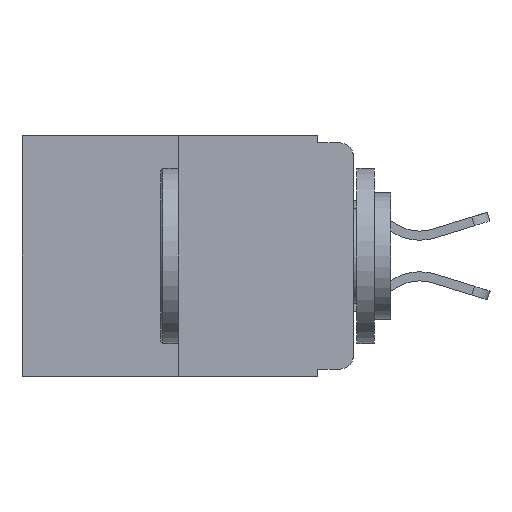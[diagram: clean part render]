
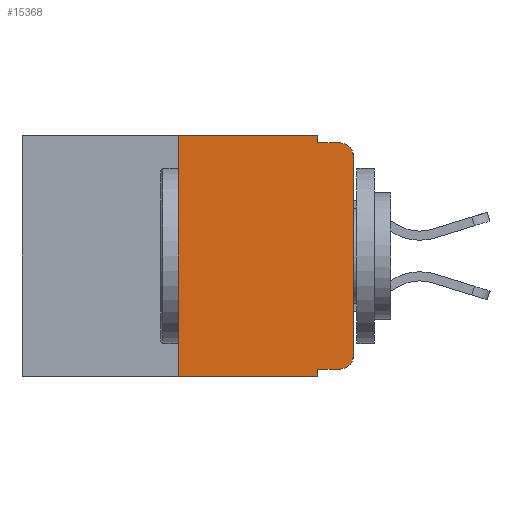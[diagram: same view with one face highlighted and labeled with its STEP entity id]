
A CAD part, left-side view. The second image highlights one B-rep face of the part: STEP entity #15368.
In plain terms, the highlighted planar face has unit normal (-1, 0, 0).
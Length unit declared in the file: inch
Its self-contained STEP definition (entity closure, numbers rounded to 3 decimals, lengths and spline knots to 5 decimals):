
#234 = ORIENTED_EDGE ( 'NONE', *, *, #13772, .T. ) ;
#562 = CARTESIAN_POINT ( 'NONE',  ( 0., 0.02, -0.03 ) ) ;
#959 = ORIENTED_EDGE ( 'NONE', *, *, #2726, .T. ) ;
#1015 = ORIENTED_EDGE ( 'NONE', *, *, #2249, .F. ) ;
#1059 = LINE ( 'NONE', #11792, #5077 ) ;
#1113 = CARTESIAN_POINT ( 'NONE',  ( 0., 0.25, 0. ) ) ;
#1494 = EDGE_LOOP ( 'NONE', ( #15183, #959, #10539, #1015, #7607, #7283, #234, #2650, #3972, #12098 ) ) ;
#1776 = VECTOR ( 'NONE', #1814, 39.37008 ) ;
#1783 = CARTESIAN_POINT ( 'NONE',  ( 0., 0.25, 0. ) ) ;
#1814 = DIRECTION ( 'NONE',  ( 0., 0., -1. ) ) ;
#2084 = LINE ( 'NONE', #13075, #10137 ) ;
#2249 = EDGE_CURVE ( 'NONE', #5030, #8816, #14380, .T. ) ;
#2281 = AXIS2_PLACEMENT_3D ( 'NONE', #12728, #11299, #8913 ) ;
#2309 = VERTEX_POINT ( 'NONE', #2767 ) ;
#2650 = ORIENTED_EDGE ( 'NONE', *, *, #3902, .F. ) ;
#2726 = EDGE_CURVE ( 'NONE', #13421, #11407, #7507, .T. ) ;
#2767 = CARTESIAN_POINT ( 'NONE',  ( 0., 0.25, -0.343 ) ) ;
#2811 = CARTESIAN_POINT ( 'NONE',  ( 0., 0., -0.03 ) ) ;
#2912 = CARTESIAN_POINT ( 'NONE',  ( 0., 0., -0.313 ) ) ;
#3123 = VERTEX_POINT ( 'NONE', #8086 ) ;
#3195 = VECTOR ( 'NONE', #13017, 39.37008 ) ;
#3245 = CARTESIAN_POINT ( 'NONE',  ( 0., 0.051, 0. ) ) ;
#3513 = CIRCLE ( 'NONE', #2281, 0.02 ) ;
#3902 = EDGE_CURVE ( 'NONE', #3123, #12696, #7713, .T. ) ;
#3972 = ORIENTED_EDGE ( 'NONE', *, *, #10650, .T. ) ;
#3991 = EDGE_CURVE ( 'NONE', #5268, #13049, #3513, .T. ) ;
#4136 = DIRECTION ( 'NONE',  ( -1., 0., 0. ) ) ;
#4153 = CARTESIAN_POINT ( 'NONE',  ( 0., 0.051, 0. ) ) ;
#4426 = CARTESIAN_POINT ( 'NONE',  ( 0., 0.473, -0.343 ) ) ;
#4637 = DIRECTION ( 'NONE',  ( 0., -1., 0. ) ) ;
#5030 = VERTEX_POINT ( 'NONE', #7222 ) ;
#5077 = VECTOR ( 'NONE', #4637, 39.37008 ) ;
#5268 = VERTEX_POINT ( 'NONE', #6978 ) ;
#5387 = CARTESIAN_POINT ( 'NONE',  ( 0., 0.051, -0.333 ) ) ;
#5455 = LINE ( 'NONE', #5387, #13763 ) ;
#5885 = DIRECTION ( 'NONE',  ( 0., 0., 1. ) ) ;
#6843 = CARTESIAN_POINT ( 'NONE',  ( 0., 0.051, -0.343 ) ) ;
#6978 = CARTESIAN_POINT ( 'NONE',  ( 0., 0.02, -0.333 ) ) ;
#7222 = CARTESIAN_POINT ( 'NONE',  ( 0., 0.051, 0. ) ) ;
#7283 = ORIENTED_EDGE ( 'NONE', *, *, #11773, .F. ) ;
#7507 = CIRCLE ( 'NONE', #9038, 0.02 ) ;
#7607 = ORIENTED_EDGE ( 'NONE', *, *, #8214, .F. ) ;
#7713 = LINE ( 'NONE', #4153, #1776 ) ;
#7765 = DIRECTION ( 'NONE',  ( 0., -1., 0. ) ) ;
#8025 = DIRECTION ( 'NONE',  ( 0., -1., 0. ) ) ;
#8056 = VERTEX_POINT ( 'NONE', #1783 ) ;
#8086 = CARTESIAN_POINT ( 'NONE',  ( 0., 0.051, -0.333 ) ) ;
#8108 = AXIS2_PLACEMENT_3D ( 'NONE', #8296, #13148, #10676 ) ;
#8214 = EDGE_CURVE ( 'NONE', #8056, #5030, #1059, .T. ) ;
#8296 = CARTESIAN_POINT ( 'NONE',  ( 0., 0.473, 0. ) ) ;
#8583 = CARTESIAN_POINT ( 'NONE',  ( 0., 0.051, -0.01 ) ) ;
#8816 = VERTEX_POINT ( 'NONE', #8583 ) ;
#8913 = DIRECTION ( 'NONE',  ( 0., 0., -1. ) ) ;
#8967 = VECTOR ( 'NONE', #5885, 39.37008 ) ;
#8972 = DIRECTION ( 'NONE',  ( 0., 0., -1. ) ) ;
#9038 = AXIS2_PLACEMENT_3D ( 'NONE', #562, #4136, #8972 ) ;
#9222 = LINE ( 'NONE', #10093, #14747 ) ;
#9341 = LINE ( 'NONE', #4426, #3195 ) ;
#10093 = CARTESIAN_POINT ( 'NONE',  ( 0., 0.051, -0.01 ) ) ;
#10137 = VECTOR ( 'NONE', #11710, 39.37008 ) ;
#10226 = EDGE_CURVE ( 'NONE', #8816, #11407, #9222, .T. ) ;
#10539 = ORIENTED_EDGE ( 'NONE', *, *, #10226, .F. ) ;
#10545 = VECTOR ( 'NONE', #12899, 39.37008 ) ;
#10588 = PLANE ( 'NONE',  #8108 ) ;
#10650 = EDGE_CURVE ( 'NONE', #3123, #5268, #5455, .T. ) ;
#10676 = DIRECTION ( 'NONE',  ( 0., 0., -1. ) ) ;
#10833 = CARTESIAN_POINT ( 'NONE',  ( 0., 0.02, -0.01 ) ) ;
#11299 = DIRECTION ( 'NONE',  ( -1., 0., 0. ) ) ;
#11407 = VERTEX_POINT ( 'NONE', #10833 ) ;
#11710 = DIRECTION ( 'NONE',  ( 0., 0., 1. ) ) ;
#11773 = EDGE_CURVE ( 'NONE', #2309, #8056, #11916, .T. ) ;
#11792 = CARTESIAN_POINT ( 'NONE',  ( 0., 0.473, 0. ) ) ;
#11916 = LINE ( 'NONE', #1113, #8967 ) ;
#12098 = ORIENTED_EDGE ( 'NONE', *, *, #3991, .T. ) ;
#12696 = VERTEX_POINT ( 'NONE', #6843 ) ;
#12728 = CARTESIAN_POINT ( 'NONE',  ( 0., 0.02, -0.313 ) ) ;
#12899 = DIRECTION ( 'NONE',  ( 0., 0., -1. ) ) ;
#13017 = DIRECTION ( 'NONE',  ( 0., -1., 0. ) ) ;
#13049 = VERTEX_POINT ( 'NONE', #2912 ) ;
#13075 = CARTESIAN_POINT ( 'NONE',  ( 0., 0., 0. ) ) ;
#13148 = DIRECTION ( 'NONE',  ( 1., 0., 0. ) ) ;
#13229 = FACE_OUTER_BOUND ( 'NONE', #1494, .T. ) ;
#13421 = VERTEX_POINT ( 'NONE', #2811 ) ;
#13763 = VECTOR ( 'NONE', #7765, 39.37008 ) ;
#13772 = EDGE_CURVE ( 'NONE', #2309, #12696, #9341, .T. ) ;
#14380 = LINE ( 'NONE', #3245, #10545 ) ;
#14747 = VECTOR ( 'NONE', #8025, 39.37008 ) ;
#15183 = ORIENTED_EDGE ( 'NONE', *, *, #15413, .T. ) ;
#15368 = ADVANCED_FACE ( 'NONE', ( #13229 ), #10588, .F. ) ;
#15413 = EDGE_CURVE ( 'NONE', #13049, #13421, #2084, .T. ) ;
